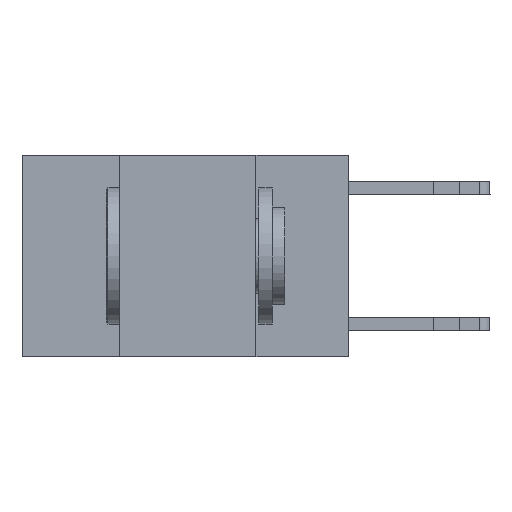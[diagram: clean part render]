
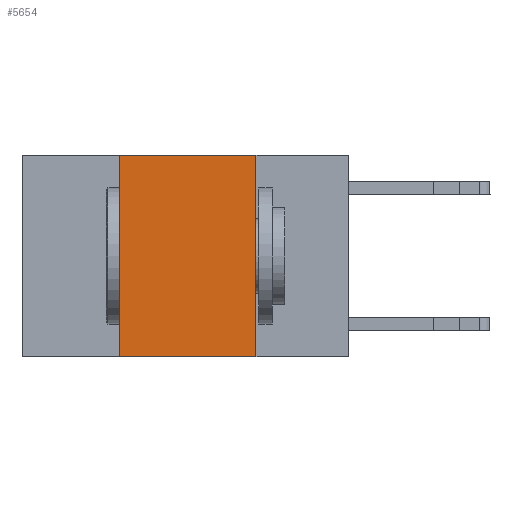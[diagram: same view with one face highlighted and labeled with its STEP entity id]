
A CAD part, left-side view. The second image highlights one B-rep face of the part: STEP entity #5654.
In plain terms, the highlighted planar face has unit normal (-1, 0, 0).
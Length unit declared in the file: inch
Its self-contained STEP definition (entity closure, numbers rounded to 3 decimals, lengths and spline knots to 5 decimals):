
#1670 = EDGE_CURVE ( 'NONE', #11670, #3530, #10222, .T. ) ;
#1797 = EDGE_CURVE ( 'NONE', #2872, #3530, #4799, .T. ) ;
#2740 = PLANE ( 'NONE',  #4779 ) ;
#2831 = CARTESIAN_POINT ( 'NONE',  ( 0., 0.6, 0. ) ) ;
#2872 = VERTEX_POINT ( 'NONE', #13463 ) ;
#3246 = CARTESIAN_POINT ( 'NONE',  ( 0., 0.42, 0. ) ) ;
#3530 = VERTEX_POINT ( 'NONE', #5523 ) ;
#4224 = CARTESIAN_POINT ( 'NONE',  ( 0., 0.6, 0. ) ) ;
#4779 = AXIS2_PLACEMENT_3D ( 'NONE', #2831, #8537, #15834 ) ;
#4799 = LINE ( 'NONE', #16675, #12431 ) ;
#4936 = LINE ( 'NONE', #3246, #6165 ) ;
#5523 = CARTESIAN_POINT ( 'NONE',  ( 0., 0.17, -0.37 ) ) ;
#5654 = ADVANCED_FACE ( 'NONE', ( #8731 ), #2740, .F. ) ;
#6041 = CARTESIAN_POINT ( 'NONE',  ( 0., 0.17, 0. ) ) ;
#6165 = VECTOR ( 'NONE', #17743, 39.37008 ) ;
#6324 = DIRECTION ( 'NONE',  ( 0., -1., 0. ) ) ;
#6720 = CARTESIAN_POINT ( 'NONE',  ( 0., 0.17, 0. ) ) ;
#7264 = LINE ( 'NONE', #4224, #17688 ) ;
#8231 = ORIENTED_EDGE ( 'NONE', *, *, #1797, .T. ) ;
#8537 = DIRECTION ( 'NONE',  ( 1., 0., 0. ) ) ;
#8715 = ORIENTED_EDGE ( 'NONE', *, *, #13758, .F. ) ;
#8731 = FACE_OUTER_BOUND ( 'NONE', #15446, .T. ) ;
#9464 = CARTESIAN_POINT ( 'NONE',  ( 0., 0.42, 0. ) ) ;
#9847 = EDGE_CURVE ( 'NONE', #2872, #18366, #4936, .T. ) ;
#9862 = ORIENTED_EDGE ( 'NONE', *, *, #1670, .F. ) ;
#10222 = LINE ( 'NONE', #6041, #16346 ) ;
#11670 = VERTEX_POINT ( 'NONE', #6720 ) ;
#12065 = ORIENTED_EDGE ( 'NONE', *, *, #9847, .F. ) ;
#12431 = VECTOR ( 'NONE', #6324, 39.37008 ) ;
#13463 = CARTESIAN_POINT ( 'NONE',  ( 0., 0.42, -0.37 ) ) ;
#13758 = EDGE_CURVE ( 'NONE', #18366, #11670, #7264, .T. ) ;
#14219 = DIRECTION ( 'NONE',  ( 0., -1., 0. ) ) ;
#14592 = DIRECTION ( 'NONE',  ( 0., 0., -1. ) ) ;
#15446 = EDGE_LOOP ( 'NONE', ( #9862, #8715, #12065, #8231 ) ) ;
#15834 = DIRECTION ( 'NONE',  ( 0., 0., -1. ) ) ;
#16346 = VECTOR ( 'NONE', #14592, 39.37008 ) ;
#16675 = CARTESIAN_POINT ( 'NONE',  ( 0., 0.6, -0.37 ) ) ;
#17688 = VECTOR ( 'NONE', #14219, 39.37008 ) ;
#17743 = DIRECTION ( 'NONE',  ( 0., 0., 1. ) ) ;
#18366 = VERTEX_POINT ( 'NONE', #9464 ) ;
